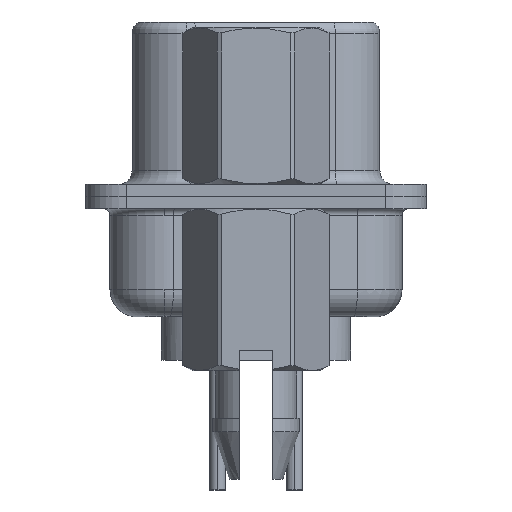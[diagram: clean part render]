
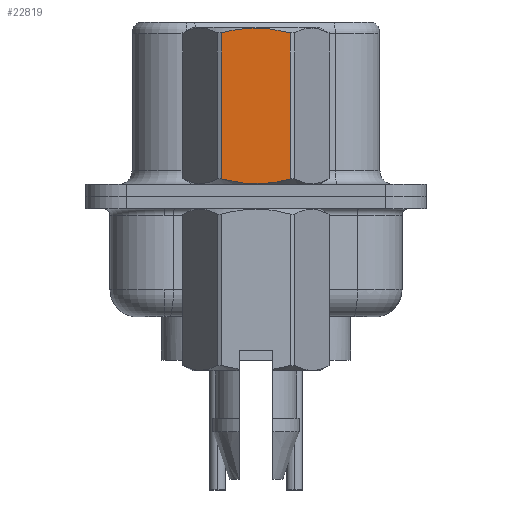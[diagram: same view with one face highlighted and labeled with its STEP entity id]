
A CAD part, left-side view. The second image highlights one B-rep face of the part: STEP entity #22819.
In plain terms, the highlighted planar face has unit normal (-1, 0, 0).
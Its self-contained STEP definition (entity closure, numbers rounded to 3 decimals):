
#294 = DIRECTION ( 'NONE',  ( 0., 0., -1. ) ) ;
#366 = CARTESIAN_POINT ( 'NONE',  ( -2.381, 1.065, 6.104 ) ) ;
#689 = CARTESIAN_POINT ( 'NONE',  ( -2.381, -1.273, 0.652 ) ) ;
#796 = CARTESIAN_POINT ( 'NONE',  ( -2.381, 1.273, 0.652 ) ) ;
#1462 = CARTESIAN_POINT ( 'NONE',  ( -2.381, -0.432, 0.485 ) ) ;
#2872 = CARTESIAN_POINT ( 'NONE',  ( -2.381, 0.215, 6.232 ) ) ;
#3182 = CARTESIAN_POINT ( 'NONE',  ( -2.381, -1.273, 6.048 ) ) ;
#4012 = ORIENTED_EDGE ( 'NONE', *, *, #12181, .T. ) ;
#5335 = B_SPLINE_CURVE_WITH_KNOTS ( 'NONE', 3,
 ( #20824, #27886, #18467, #6173, #11044, #18316, #1462, #20665, #25515, #23175 ),
 .UNSPECIFIED., .F., .F.,
 ( 4, 2, 2, 2, 4 ),
 ( 0.003, 0.003, 0.004, 0.004, 0.005 ),
 .UNSPECIFIED. ) ;
#5377 = VERTEX_POINT ( 'NONE', #689 ) ;
#6173 = CARTESIAN_POINT ( 'NONE',  ( -2.381, 0.428, 0.485 ) ) ;
#7756 = CARTESIAN_POINT ( 'NONE',  ( -2.381, 1.375, -3.75 ) ) ;
#7902 = CARTESIAN_POINT ( 'NONE',  ( -2.381, 0.428, 6.215 ) ) ;
#7981 = CARTESIAN_POINT ( 'NONE',  ( -2.381, 1.273, 3.792 ) ) ;
#10099 = DIRECTION ( 'NONE',  ( -1., 0., 0. ) ) ;
#11044 = CARTESIAN_POINT ( 'NONE',  ( -2.381, 0.215, 0.468 ) ) ;
#11739 = VERTEX_POINT ( 'NONE', #24299 ) ;
#12181 = EDGE_CURVE ( 'NONE', #16305, #5377, #5335, .T. ) ;
#13711 = VECTOR ( 'NONE', #294, 1000. ) ;
#14287 = ORIENTED_EDGE ( 'NONE', *, *, #25441, .T. ) ;
#14522 = DIRECTION ( 'NONE',  ( 0., -1., 0. ) ) ;
#14851 = CARTESIAN_POINT ( 'NONE',  ( -2.381, -0.858, 6.15 ) ) ;
#16305 = VERTEX_POINT ( 'NONE', #796 ) ;
#17051 = CARTESIAN_POINT ( 'NONE',  ( -2.381, 1.273, 6.048 ) ) ;
#18316 = CARTESIAN_POINT ( 'NONE',  ( -2.381, -0.215, 0.468 ) ) ;
#18467 = CARTESIAN_POINT ( 'NONE',  ( -2.381, 0.853, 0.549 ) ) ;
#19699 = LINE ( 'NONE', #28950, #27682 ) ;
#19854 = DIRECTION ( 'NONE',  ( 0., 0., 1. ) ) ;
#19892 = CARTESIAN_POINT ( 'NONE',  ( -2.381, -0.432, 6.215 ) ) ;
#20665 = CARTESIAN_POINT ( 'NONE',  ( -2.381, -0.858, 0.55 ) ) ;
#20824 = CARTESIAN_POINT ( 'NONE',  ( -2.381, 1.273, 0.652 ) ) ;
#22318 = LINE ( 'NONE', #7981, #13711 ) ;
#22355 = CARTESIAN_POINT ( 'NONE',  ( -2.381, -1.273, 6.048 ) ) ;
#22819 = ADVANCED_FACE ( 'NONE', ( #26469 ), #28985, .T. ) ;
#23175 = CARTESIAN_POINT ( 'NONE',  ( -2.381, -1.273, 0.652 ) ) ;
#24120 = CARTESIAN_POINT ( 'NONE',  ( -2.381, -1.066, 6.104 ) ) ;
#24299 = CARTESIAN_POINT ( 'NONE',  ( -2.381, 1.273, 6.048 ) ) ;
#25047 = EDGE_CURVE ( 'NONE', #25445, #11739, #27331, .T. ) ;
#25346 = ORIENTED_EDGE ( 'NONE', *, *, #28883, .T. ) ;
#25441 = EDGE_CURVE ( 'NONE', #5377, #25445, #19699, .T. ) ;
#25445 = VERTEX_POINT ( 'NONE', #22355 ) ;
#25515 = CARTESIAN_POINT ( 'NONE',  ( -2.381, -1.066, 0.596 ) ) ;
#26469 = FACE_OUTER_BOUND ( 'NONE', #29240, .T. ) ;
#27093 = CARTESIAN_POINT ( 'NONE',  ( -2.381, -0.215, 6.232 ) ) ;
#27331 = B_SPLINE_CURVE_WITH_KNOTS ( 'NONE', 3,
 ( #3182, #24120, #14851, #19892, #27093, #2872, #7902, #28987, #366, #17051 ),
 .UNSPECIFIED., .F., .F.,
 ( 4, 2, 2, 2, 4 ),
 ( 0.001, 0.002, 0.002, 0.003, 0.004 ),
 .UNSPECIFIED. ) ;
#27572 = AXIS2_PLACEMENT_3D ( 'NONE', #7756, #10099, #14522 ) ;
#27682 = VECTOR ( 'NONE', #19854, 1000. ) ;
#27881 = ORIENTED_EDGE ( 'NONE', *, *, #25047, .T. ) ;
#27886 = CARTESIAN_POINT ( 'NONE',  ( -2.381, 1.065, 0.596 ) ) ;
#28883 = EDGE_CURVE ( 'NONE', #11739, #16305, #22318, .T. ) ;
#28950 = CARTESIAN_POINT ( 'NONE',  ( -2.381, -1.273, 3.792 ) ) ;
#28985 = PLANE ( 'NONE',  #27572 ) ;
#28987 = CARTESIAN_POINT ( 'NONE',  ( -2.381, 0.853, 6.151 ) ) ;
#29240 = EDGE_LOOP ( 'NONE', ( #4012, #14287, #27881, #25346 ) ) ;
